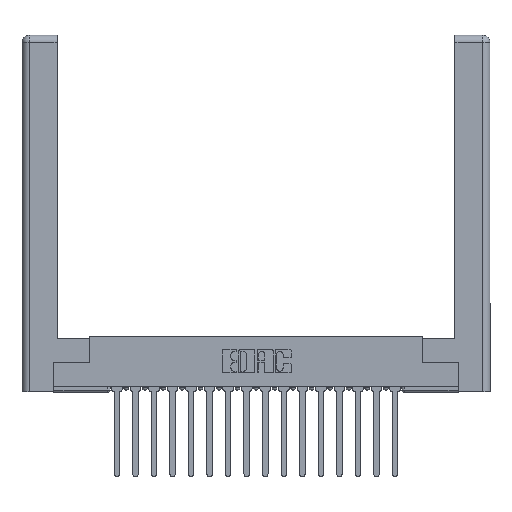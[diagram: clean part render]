
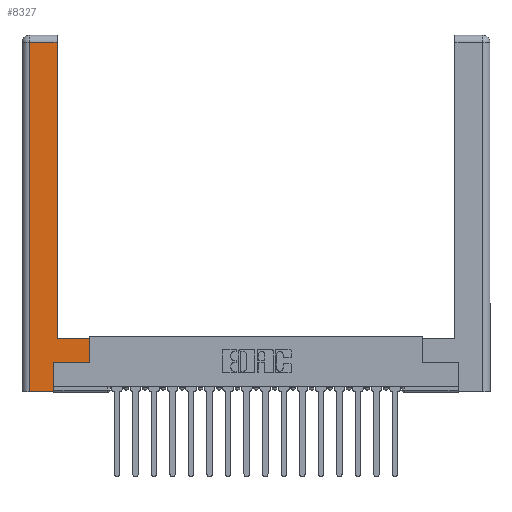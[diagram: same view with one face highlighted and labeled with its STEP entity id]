
A CAD part, top view. The second image highlights one B-rep face of the part: STEP entity #8327.
In plain terms, the highlighted planar face has unit normal (0, 0, 1).
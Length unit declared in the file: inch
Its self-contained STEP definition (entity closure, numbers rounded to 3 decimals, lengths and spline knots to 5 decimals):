
#193 = EDGE_CURVE ( 'NONE', #3490, #11796, #13790, .T. ) ;
#264 = LINE ( 'NONE', #8896, #6781 ) ;
#742 = VECTOR ( 'NONE', #9268, 39.37008 ) ;
#890 = VECTOR ( 'NONE', #7207, 39.37008 ) ;
#1170 = LINE ( 'NONE', #19488, #18856 ) ;
#1394 = EDGE_CURVE ( 'NONE', #5805, #2832, #1170, .T. ) ;
#1437 = DIRECTION ( 'NONE',  ( -1., 0., 0. ) ) ;
#1751 = DIRECTION ( 'NONE',  ( 0., 1., 0. ) ) ;
#1799 = EDGE_CURVE ( 'NONE', #8263, #3490, #2348, .T. ) ;
#1811 = VECTOR ( 'NONE', #1751, 39.37008 ) ;
#1997 = EDGE_LOOP ( 'NONE', ( #2275, #9720, #12442, #3904, #15512, #9354, #13361, #2959 ) ) ;
#2275 = ORIENTED_EDGE ( 'NONE', *, *, #13681, .T. ) ;
#2348 = LINE ( 'NONE', #13074, #3818 ) ;
#2832 = VERTEX_POINT ( 'NONE', #4309 ) ;
#2959 = ORIENTED_EDGE ( 'NONE', *, *, #193, .T. ) ;
#3490 = VERTEX_POINT ( 'NONE', #19709 ) ;
#3818 = VECTOR ( 'NONE', #13003, 39.37008 ) ;
#3904 = ORIENTED_EDGE ( 'NONE', *, *, #18621, .T. ) ;
#3974 = LINE ( 'NONE', #7911, #1811 ) ;
#4273 = CARTESIAN_POINT ( 'NONE',  ( 0.295, 2.94, 0. ) ) ;
#4309 = CARTESIAN_POINT ( 'NONE',  ( 0.265, 0.245, 0. ) ) ;
#4670 = AXIS2_PLACEMENT_3D ( 'NONE', #6395, #17130, #17201 ) ;
#5215 = CARTESIAN_POINT ( 'NONE',  ( 0.295, 0.45, 0. ) ) ;
#5650 = FACE_OUTER_BOUND ( 'NONE', #1997, .T. ) ;
#5737 = VERTEX_POINT ( 'NONE', #16888 ) ;
#5805 = VERTEX_POINT ( 'NONE', #6210 ) ;
#6210 = CARTESIAN_POINT ( 'NONE',  ( 0.265, 0., 0. ) ) ;
#6395 = CARTESIAN_POINT ( 'NONE',  ( 0., 0., 0. ) ) ;
#6781 = VECTOR ( 'NONE', #7477, 39.37008 ) ;
#7207 = DIRECTION ( 'NONE',  ( 1., 0., 0. ) ) ;
#7466 = CARTESIAN_POINT ( 'NONE',  ( 0.0615, 2.94, 0. ) ) ;
#7477 = DIRECTION ( 'NONE',  ( 0., -1., 0. ) ) ;
#7841 = VECTOR ( 'NONE', #15101, 39.37008 ) ;
#7911 = CARTESIAN_POINT ( 'NONE',  ( 0.295, 3., 0. ) ) ;
#8263 = VERTEX_POINT ( 'NONE', #15154 ) ;
#8327 = ADVANCED_FACE ( 'NONE', ( #5650 ), #9365, .F. ) ;
#8770 = VERTEX_POINT ( 'NONE', #4273 ) ;
#8896 = CARTESIAN_POINT ( 'NONE',  ( 0.0615, 0., 0. ) ) ;
#8912 = CARTESIAN_POINT ( 'NONE',  ( 0.565, 0.245, 0. ) ) ;
#9202 = VERTEX_POINT ( 'NONE', #14579 ) ;
#9268 = DIRECTION ( 'NONE',  ( -1., 0., 0. ) ) ;
#9354 = ORIENTED_EDGE ( 'NONE', *, *, #14066, .T. ) ;
#9365 = PLANE ( 'NONE',  #4670 ) ;
#9720 = ORIENTED_EDGE ( 'NONE', *, *, #14707, .T. ) ;
#10249 = LINE ( 'NONE', #7466, #17740 ) ;
#10340 = LINE ( 'NONE', #13544, #890 ) ;
#10755 = DIRECTION ( 'NONE',  ( 0., 1., 0. ) ) ;
#11796 = VERTEX_POINT ( 'NONE', #5215 ) ;
#12442 = ORIENTED_EDGE ( 'NONE', *, *, #16802, .T. ) ;
#13003 = DIRECTION ( 'NONE',  ( 0., 1., 0. ) ) ;
#13074 = CARTESIAN_POINT ( 'NONE',  ( 0.565, 0.45, 0. ) ) ;
#13361 = ORIENTED_EDGE ( 'NONE', *, *, #1799, .T. ) ;
#13544 = CARTESIAN_POINT ( 'NONE',  ( 0.265, 0., 0. ) ) ;
#13681 = EDGE_CURVE ( 'NONE', #11796, #8770, #3974, .T. ) ;
#13790 = LINE ( 'NONE', #14286, #742 ) ;
#14066 = EDGE_CURVE ( 'NONE', #2832, #8263, #18983, .T. ) ;
#14286 = CARTESIAN_POINT ( 'NONE',  ( 0.295, 0.45, 0. ) ) ;
#14579 = CARTESIAN_POINT ( 'NONE',  ( 0.0615, 2.94, 0. ) ) ;
#14707 = EDGE_CURVE ( 'NONE', #8770, #9202, #10249, .T. ) ;
#15101 = DIRECTION ( 'NONE',  ( 1., 0., 0. ) ) ;
#15154 = CARTESIAN_POINT ( 'NONE',  ( 0.565, 0.245, 0. ) ) ;
#15512 = ORIENTED_EDGE ( 'NONE', *, *, #1394, .T. ) ;
#16802 = EDGE_CURVE ( 'NONE', #9202, #5737, #264, .T. ) ;
#16888 = CARTESIAN_POINT ( 'NONE',  ( 0.0615, 0., 0. ) ) ;
#17130 = DIRECTION ( 'NONE',  ( 0., 0., -1. ) ) ;
#17201 = DIRECTION ( 'NONE',  ( -1., 0., 0. ) ) ;
#17740 = VECTOR ( 'NONE', #1437, 39.37008 ) ;
#18621 = EDGE_CURVE ( 'NONE', #5737, #5805, #10340, .T. ) ;
#18856 = VECTOR ( 'NONE', #10755, 39.37008 ) ;
#18983 = LINE ( 'NONE', #8912, #7841 ) ;
#19488 = CARTESIAN_POINT ( 'NONE',  ( 0.265, 0.245, 0. ) ) ;
#19709 = CARTESIAN_POINT ( 'NONE',  ( 0.565, 0.45, 0. ) ) ;
